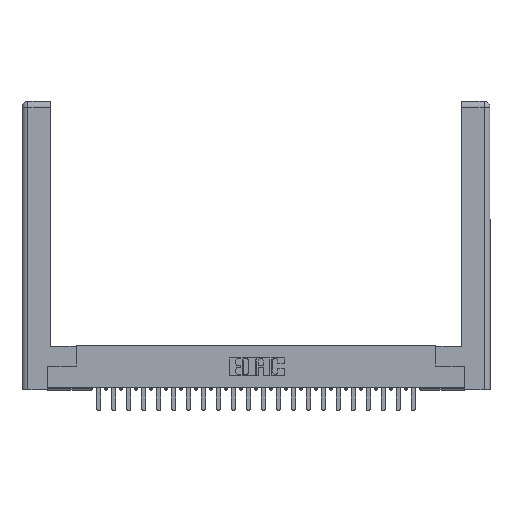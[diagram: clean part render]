
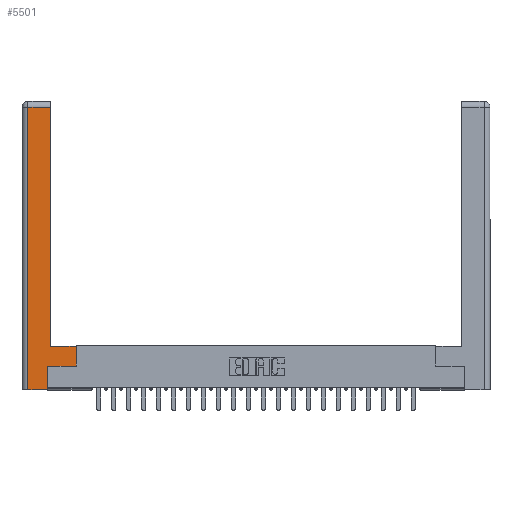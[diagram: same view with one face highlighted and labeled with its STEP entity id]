
A CAD part, top view. The second image highlights one B-rep face of the part: STEP entity #5501.
In plain terms, the highlighted planar face has unit normal (0, 0, 1).
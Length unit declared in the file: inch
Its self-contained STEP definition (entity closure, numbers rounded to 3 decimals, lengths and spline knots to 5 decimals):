
#478 = LINE ( 'NONE', #15826, #8722 ) ;
#581 = VERTEX_POINT ( 'NONE', #2685 ) ;
#810 = ORIENTED_EDGE ( 'NONE', *, *, #3783, .T. ) ;
#1631 = ORIENTED_EDGE ( 'NONE', *, *, #5666, .T. ) ;
#2685 = CARTESIAN_POINT ( 'NONE',  ( 0.265, 0.245, 0. ) ) ;
#2781 = PLANE ( 'NONE',  #8911 ) ;
#3077 = LINE ( 'NONE', #6644, #22516 ) ;
#3439 = CARTESIAN_POINT ( 'NONE',  ( 0.295, 0.45, 0. ) ) ;
#3633 = VERTEX_POINT ( 'NONE', #13749 ) ;
#3783 = EDGE_CURVE ( 'NONE', #24591, #21663, #13761, .T. ) ;
#3902 = VECTOR ( 'NONE', #22773, 39.37008 ) ;
#3949 = VERTEX_POINT ( 'NONE', #26284 ) ;
#4111 = DIRECTION ( 'NONE',  ( 0., 1., 0. ) ) ;
#4420 = VERTEX_POINT ( 'NONE', #26323 ) ;
#4584 = VECTOR ( 'NONE', #14367, 39.37008 ) ;
#4684 = DIRECTION ( 'NONE',  ( 1., 0., 0. ) ) ;
#5501 = ADVANCED_FACE ( 'NONE', ( #16450 ), #2781, .F. ) ;
#5666 = EDGE_CURVE ( 'NONE', #24001, #24591, #11266, .T. ) ;
#5726 = CARTESIAN_POINT ( 'NONE',  ( 0.265, 0., 0. ) ) ;
#5848 = ORIENTED_EDGE ( 'NONE', *, *, #16368, .T. ) ;
#6450 = VECTOR ( 'NONE', #12322, 39.37008 ) ;
#6644 = CARTESIAN_POINT ( 'NONE',  ( 0.0615, 0., 0. ) ) ;
#6883 = CARTESIAN_POINT ( 'NONE',  ( 0.295, 0.45, 0. ) ) ;
#7592 = EDGE_CURVE ( 'NONE', #27800, #4420, #478, .T. ) ;
#8112 = LINE ( 'NONE', #5726, #6450 ) ;
#8722 = VECTOR ( 'NONE', #13577, 39.37008 ) ;
#8911 = AXIS2_PLACEMENT_3D ( 'NONE', #27164, #16143, #13699 ) ;
#9266 = ORIENTED_EDGE ( 'NONE', *, *, #7592, .T. ) ;
#10181 = CARTESIAN_POINT ( 'NONE',  ( 0.265, 0.245, 0. ) ) ;
#10434 = LINE ( 'NONE', #10181, #4584 ) ;
#11266 = LINE ( 'NONE', #28787, #19566 ) ;
#11576 = CARTESIAN_POINT ( 'NONE',  ( 0.565, 0.245, 0. ) ) ;
#11694 = EDGE_CURVE ( 'NONE', #3949, #3633, #8112, .T. ) ;
#12322 = DIRECTION ( 'NONE',  ( 1., 0., 0. ) ) ;
#13577 = DIRECTION ( 'NONE',  ( -1., 0., 0. ) ) ;
#13699 = DIRECTION ( 'NONE',  ( -1., 0., 0. ) ) ;
#13749 = CARTESIAN_POINT ( 'NONE',  ( 0.265, 0., 0. ) ) ;
#13761 = LINE ( 'NONE', #3439, #27722 ) ;
#14367 = DIRECTION ( 'NONE',  ( 0., 1., 0. ) ) ;
#15826 = CARTESIAN_POINT ( 'NONE',  ( 0.0615, 2.94, 0. ) ) ;
#16143 = DIRECTION ( 'NONE',  ( 0., 0., -1. ) ) ;
#16368 = EDGE_CURVE ( 'NONE', #581, #24001, #26630, .T. ) ;
#16450 = FACE_OUTER_BOUND ( 'NONE', #24372, .T. ) ;
#17435 = CARTESIAN_POINT ( 'NONE',  ( 0.295, 2.94, 0. ) ) ;
#18662 = ORIENTED_EDGE ( 'NONE', *, *, #23704, .T. ) ;
#19566 = VECTOR ( 'NONE', #4111, 39.37008 ) ;
#21663 = VERTEX_POINT ( 'NONE', #6883 ) ;
#22507 = CARTESIAN_POINT ( 'NONE',  ( 0.565, 0.245, 0. ) ) ;
#22516 = VECTOR ( 'NONE', #28654, 39.37008 ) ;
#22727 = VECTOR ( 'NONE', #4684, 39.37008 ) ;
#22773 = DIRECTION ( 'NONE',  ( 0., 1., 0. ) ) ;
#22930 = ORIENTED_EDGE ( 'NONE', *, *, #25987, .T. ) ;
#23704 = EDGE_CURVE ( 'NONE', #3633, #581, #10434, .T. ) ;
#24001 = VERTEX_POINT ( 'NONE', #11576 ) ;
#24372 = EDGE_LOOP ( 'NONE', ( #25923, #9266, #22930, #28005, #18662, #5848, #1631, #810 ) ) ;
#24591 = VERTEX_POINT ( 'NONE', #25498 ) ;
#25429 = LINE ( 'NONE', #27971, #3902 ) ;
#25498 = CARTESIAN_POINT ( 'NONE',  ( 0.565, 0.45, 0. ) ) ;
#25923 = ORIENTED_EDGE ( 'NONE', *, *, #26679, .T. ) ;
#25987 = EDGE_CURVE ( 'NONE', #4420, #3949, #3077, .T. ) ;
#26284 = CARTESIAN_POINT ( 'NONE',  ( 0.0615, 0., 0. ) ) ;
#26323 = CARTESIAN_POINT ( 'NONE',  ( 0.0615, 2.94, 0. ) ) ;
#26630 = LINE ( 'NONE', #22507, #22727 ) ;
#26679 = EDGE_CURVE ( 'NONE', #21663, #27800, #25429, .T. ) ;
#27164 = CARTESIAN_POINT ( 'NONE',  ( 0., 0., 0. ) ) ;
#27722 = VECTOR ( 'NONE', #27831, 39.37008 ) ;
#27800 = VERTEX_POINT ( 'NONE', #17435 ) ;
#27831 = DIRECTION ( 'NONE',  ( -1., 0., 0. ) ) ;
#27971 = CARTESIAN_POINT ( 'NONE',  ( 0.295, 3., 0. ) ) ;
#28005 = ORIENTED_EDGE ( 'NONE', *, *, #11694, .T. ) ;
#28654 = DIRECTION ( 'NONE',  ( 0., -1., 0. ) ) ;
#28787 = CARTESIAN_POINT ( 'NONE',  ( 0.565, 0.45, 0. ) ) ;
